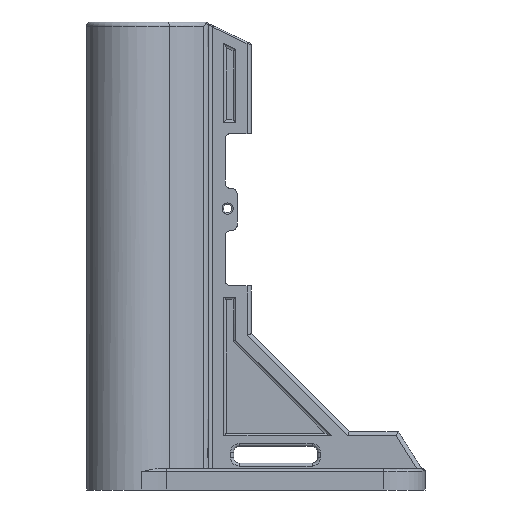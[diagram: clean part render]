
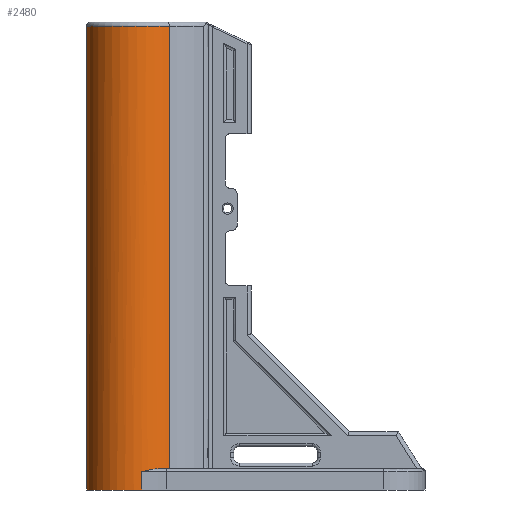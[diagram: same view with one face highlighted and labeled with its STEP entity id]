
A CAD part, left-side view. The second image highlights one B-rep face of the part: STEP entity #2480.
In plain terms, the highlighted cylindrical face has radius 17.99 mm (diameter 35.98 mm), a partial arc.
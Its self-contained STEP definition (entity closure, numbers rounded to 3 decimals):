
#15=CYLINDRICAL_SURFACE('',#2658,17.99);
#152=LINE('',#3866,#357);
#153=LINE('',#3877,#358);
#154=LINE('',#3881,#359);
#155=LINE('',#3891,#360);
#357=VECTOR('',#2982,10.);
#358=VECTOR('',#2985,10.);
#359=VECTOR('',#2988,10.);
#360=VECTOR('',#2991,10.);
#617=B_SPLINE_CURVE_WITH_KNOTS('',3,(#3870,#3871,#3872,#3873,#3874,#3875),
 .UNSPECIFIED.,.F.,.F.,(4,2,4),(1.669,2.168,2.17),
 .UNSPECIFIED.);
#618=B_SPLINE_CURVE_WITH_KNOTS('',3,(#3883,#3884,#3885,#3886,#3887,#3888),
 .UNSPECIFIED.,.F.,.F.,(4,2,4),(-0.002,0.,0.66),
 .UNSPECIFIED.);
#640=FACE_OUTER_BOUND('',#790,.T.);
#790=EDGE_LOOP('',(#1734,#1735,#1736,#1737,#1738,#1739,#1740,#1741,#1742,
#1743));
#951=CIRCLE('',#2639,17.99);
#962=CIRCLE('',#2659,17.99);
#963=CIRCLE('',#2660,17.99);
#964=CIRCLE('',#2661,17.99);
#1068=VERTEX_POINT('',#3723);
#1069=VERTEX_POINT('',#3725);
#1094=VERTEX_POINT('',#3865);
#1095=VERTEX_POINT('',#3867);
#1096=VERTEX_POINT('',#3869);
#1097=VERTEX_POINT('',#3876);
#1098=VERTEX_POINT('',#3878);
#1099=VERTEX_POINT('',#3880);
#1100=VERTEX_POINT('',#3882);
#1101=VERTEX_POINT('',#3889);
#1311=EDGE_CURVE('',#1068,#1069,#951,.T.);
#1342=EDGE_CURVE('',#1094,#1068,#152,.T.);
#1343=EDGE_CURVE('',#1095,#1094,#962,.T.);
#1344=EDGE_CURVE('',#1096,#1095,#617,.F.);
#1345=EDGE_CURVE('',#1097,#1096,#153,.T.);
#1346=EDGE_CURVE('',#1097,#1098,#963,.T.);
#1347=EDGE_CURVE('',#1099,#1098,#154,.T.);
#1348=EDGE_CURVE('',#1100,#1099,#618,.F.);
#1349=EDGE_CURVE('',#1101,#1100,#964,.T.);
#1350=EDGE_CURVE('',#1069,#1101,#155,.T.);
#1734=ORIENTED_EDGE('',*,*,#1311,.F.);
#1735=ORIENTED_EDGE('',*,*,#1342,.F.);
#1736=ORIENTED_EDGE('',*,*,#1343,.F.);
#1737=ORIENTED_EDGE('',*,*,#1344,.F.);
#1738=ORIENTED_EDGE('',*,*,#1345,.F.);
#1739=ORIENTED_EDGE('',*,*,#1346,.T.);
#1740=ORIENTED_EDGE('',*,*,#1347,.F.);
#1741=ORIENTED_EDGE('',*,*,#1348,.F.);
#1742=ORIENTED_EDGE('',*,*,#1349,.F.);
#1743=ORIENTED_EDGE('',*,*,#1350,.F.);
#2480=ADVANCED_FACE('',(#640),#15,.T.);
#2639=AXIS2_PLACEMENT_3D('',#3726,#2935,#2936);
#2658=AXIS2_PLACEMENT_3D('',#3864,#2980,#2981);
#2659=AXIS2_PLACEMENT_3D('',#3868,#2983,#2984);
#2660=AXIS2_PLACEMENT_3D('',#3879,#2986,#2987);
#2661=AXIS2_PLACEMENT_3D('',#3890,#2989,#2990);
#2935=DIRECTION('center_axis',(0.,0.,1.));
#2936=DIRECTION('ref_axis',(0.,1.,0.));
#2980=DIRECTION('center_axis',(0.,0.,-1.));
#2981=DIRECTION('ref_axis',(0.,1.,0.));
#2982=DIRECTION('',(0.,0.,1.));
#2983=DIRECTION('center_axis',(0.,0.,-1.));
#2984=DIRECTION('ref_axis',(0.588,-0.809,0.));
#2985=DIRECTION('',(0.,0.,1.));
#2986=DIRECTION('center_axis',(0.,0.,1.));
#2987=DIRECTION('ref_axis',(-0.917,0.4,0.));
#2988=DIRECTION('',(0.,0.,-1.));
#2989=DIRECTION('center_axis',(0.,0.,-1.));
#2990=DIRECTION('ref_axis',(-0.917,0.4,0.));
#2991=DIRECTION('',(0.,0.,-1.));
#3723=CARTESIAN_POINT('',(13.742,13.79,173.029));
#3725=CARTESIAN_POINT('',(-13.742,13.79,173.029));
#3726=CARTESIAN_POINT('Origin',(0.,25.4,173.029));
#3864=CARTESIAN_POINT('Origin',(0.,25.4,195.005));
#3865=CARTESIAN_POINT('',(13.742,13.79,15.));
#3866=CARTESIAN_POINT('',(13.742,13.79,180.005));
#3867=CARTESIAN_POINT('',(16.52,18.277,15.));
#3868=CARTESIAN_POINT('Origin',(0.,25.4,15.));
#3869=CARTESIAN_POINT('',(17.903,23.637,14.));
#3870=CARTESIAN_POINT('Ctrl Pts',(16.52,18.277,15.));
#3871=CARTESIAN_POINT('Ctrl Pts',(17.131,19.694,15.));
#3872=CARTESIAN_POINT('Ctrl Pts',(17.691,21.499,14.55));
#3873=CARTESIAN_POINT('Ctrl Pts',(17.902,23.626,14.003));
#3874=CARTESIAN_POINT('Ctrl Pts',(17.903,23.631,14.001));
#3875=CARTESIAN_POINT('Ctrl Pts',(17.903,23.637,14.));
#3876=CARTESIAN_POINT('',(17.903,23.637,7.46));
#3877=CARTESIAN_POINT('',(17.903,23.637,182.005));
#3878=CARTESIAN_POINT('',(-17.903,23.637,7.46));
#3879=CARTESIAN_POINT('Origin',(0.,25.4,7.46));
#3880=CARTESIAN_POINT('',(-17.903,23.637,14.));
#3881=CARTESIAN_POINT('',(-17.903,23.637,182.005));
#3882=CARTESIAN_POINT('',(-16.52,18.277,15.));
#3883=CARTESIAN_POINT('Ctrl Pts',(-17.903,23.637,14.));
#3884=CARTESIAN_POINT('Ctrl Pts',(-17.903,23.631,14.001));
#3885=CARTESIAN_POINT('Ctrl Pts',(-17.902,23.626,14.003));
#3886=CARTESIAN_POINT('Ctrl Pts',(-17.691,21.499,14.55));
#3887=CARTESIAN_POINT('Ctrl Pts',(-17.131,19.694,15.));
#3888=CARTESIAN_POINT('Ctrl Pts',(-16.52,18.277,15.));
#3889=CARTESIAN_POINT('',(-13.742,13.79,15.));
#3890=CARTESIAN_POINT('Origin',(0.,25.4,15.));
#3891=CARTESIAN_POINT('',(-13.742,13.79,195.005));
